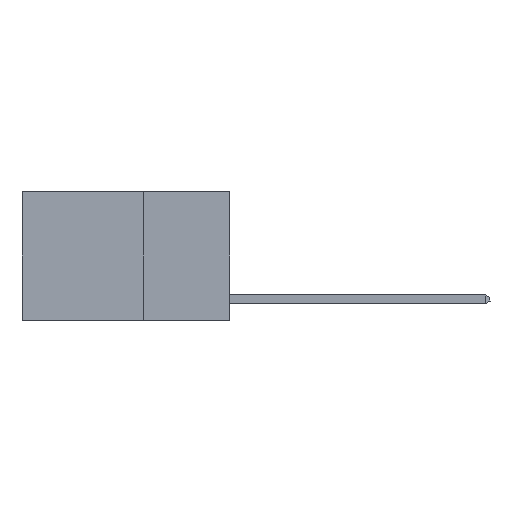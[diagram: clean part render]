
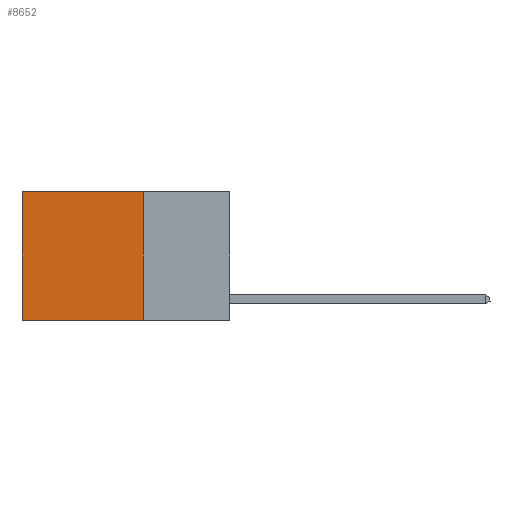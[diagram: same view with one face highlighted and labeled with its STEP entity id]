
A CAD part, left-side view. The second image highlights one B-rep face of the part: STEP entity #8652.
In plain terms, the highlighted planar face has unit normal (-1, 0, 0).
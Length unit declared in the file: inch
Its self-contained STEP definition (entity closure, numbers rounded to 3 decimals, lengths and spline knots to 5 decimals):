
#416 = CARTESIAN_POINT ( 'NONE',  ( 0.2625, 0.25, -0.37 ) ) ;
#1053 = AXIS2_PLACEMENT_3D ( 'NONE', #12110, #18693, #20382 ) ;
#1489 = VECTOR ( 'NONE', #14722, 39.37008 ) ;
#2048 = CARTESIAN_POINT ( 'NONE',  ( 0.2625, 0.25, 0. ) ) ;
#2272 = EDGE_CURVE ( 'NONE', #6224, #10178, #14202, .T. ) ;
#3342 = EDGE_CURVE ( 'NONE', #10178, #7441, #8453, .T. ) ;
#3874 = VECTOR ( 'NONE', #4518, 39.37008 ) ;
#4518 = DIRECTION ( 'NONE',  ( 0., 0., -1. ) ) ;
#4624 = CARTESIAN_POINT ( 'NONE',  ( 0.2625, 0.6, 0. ) ) ;
#5431 = VECTOR ( 'NONE', #6870, 39.37008 ) ;
#5633 = VERTEX_POINT ( 'NONE', #4624 ) ;
#5720 = PLANE ( 'NONE',  #1053 ) ;
#5843 = LINE ( 'NONE', #14051, #16842 ) ;
#6224 = VERTEX_POINT ( 'NONE', #2048 ) ;
#6870 = DIRECTION ( 'NONE',  ( 0., 1., 0. ) ) ;
#6975 = EDGE_CURVE ( 'NONE', #6224, #5633, #19379, .T. ) ;
#7441 = VERTEX_POINT ( 'NONE', #17890 ) ;
#8453 = LINE ( 'NONE', #416, #5431 ) ;
#8652 = ADVANCED_FACE ( 'NONE', ( #20278 ), #5720, .F. ) ;
#9825 = CARTESIAN_POINT ( 'NONE',  ( 0.2625, 0.25, 0. ) ) ;
#10178 = VERTEX_POINT ( 'NONE', #13488 ) ;
#11174 = ORIENTED_EDGE ( 'NONE', *, *, #2272, .F. ) ;
#12110 = CARTESIAN_POINT ( 'NONE',  ( 0.2625, 0.25, 0. ) ) ;
#13488 = CARTESIAN_POINT ( 'NONE',  ( 0.2625, 0.25, -0.37 ) ) ;
#14051 = CARTESIAN_POINT ( 'NONE',  ( 0.2625, 0.6, 0. ) ) ;
#14202 = LINE ( 'NONE', #19062, #3874 ) ;
#14722 = DIRECTION ( 'NONE',  ( 0., 1., 0. ) ) ;
#16594 = ORIENTED_EDGE ( 'NONE', *, *, #6975, .T. ) ;
#16842 = VECTOR ( 'NONE', #16913, 39.37008 ) ;
#16913 = DIRECTION ( 'NONE',  ( 0., 0., -1. ) ) ;
#16917 = EDGE_CURVE ( 'NONE', #5633, #7441, #5843, .T. ) ;
#17367 = ORIENTED_EDGE ( 'NONE', *, *, #16917, .T. ) ;
#17845 = ORIENTED_EDGE ( 'NONE', *, *, #3342, .F. ) ;
#17890 = CARTESIAN_POINT ( 'NONE',  ( 0.2625, 0.6, -0.37 ) ) ;
#18693 = DIRECTION ( 'NONE',  ( 1., 0., 0. ) ) ;
#19062 = CARTESIAN_POINT ( 'NONE',  ( 0.2625, 0.25, 0. ) ) ;
#19379 = LINE ( 'NONE', #9825, #1489 ) ;
#19566 = EDGE_LOOP ( 'NONE', ( #17367, #17845, #11174, #16594 ) ) ;
#20278 = FACE_OUTER_BOUND ( 'NONE', #19566, .T. ) ;
#20382 = DIRECTION ( 'NONE',  ( 0., 0., -1. ) ) ;
